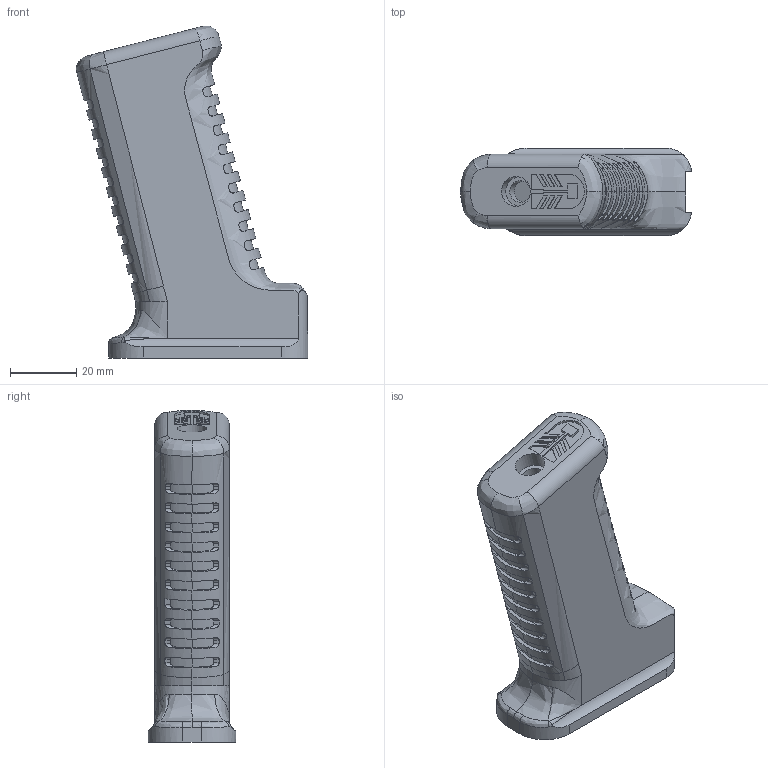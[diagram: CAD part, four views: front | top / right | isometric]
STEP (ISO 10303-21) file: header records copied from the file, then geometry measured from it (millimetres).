
FILE_DESCRIPTION(/* description */ (''),/* implementation_level */ '2;1');
FILE_NAME(/* name */ 'AK Grip Custom Final.step',/* time_stamp */ '2022-04-21T21:57:34-05:00',/* author */ (''),/* organization */ (''),/* preprocessor_version */ 'ST-DEVELOPER v18.1',/* originating_system */ 'Autodesk Translation Framework v10.14.0.1471',/* authorisation */ '');
FILE_SCHEMA (('AUTOMOTIVE_DESIGN { 1 0 10303 214 3 1 1 }'));
Length unit declared in the file: millimetre
Products named in the file (2): AK Grip Custom; Logo v1
Assembly tree (1 placements, depth 2):
  AK Grip Custom
    Logo v1
Bounding box: 69.69 x 26.5 x 100.06 mm (x, y, z)
Volume: 49621.7 mm3; surface area: 23551.3 mm2
Topology: 1 solids, 1 shells, 350 faces, 993 edges, 644 vertices
Faces by surface type: plane 179, cylinder 97, bspline 74
Full cylindrical faces by diameter (mm): 6.5 x1, 9 x1
Entity records: 20745 total; most frequent: CARTESIAN_POINT 12729, ORIENTED_EDGE 1980, DIRECTION 1134, EDGE_CURVE 990, VERTEX_POINT 644, LINE 494, VECTOR 494, B_SPLINE_CURVE_WITH_KNOTS 455
